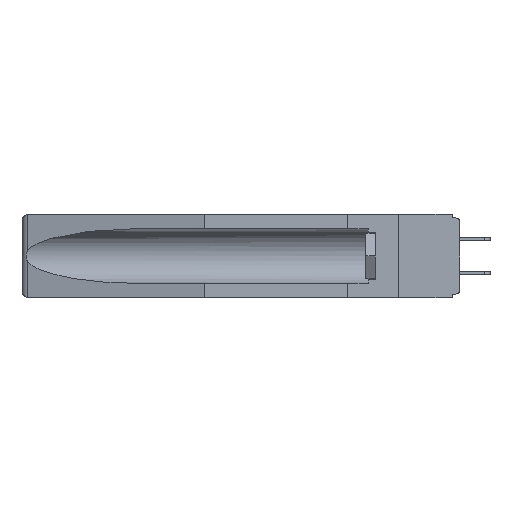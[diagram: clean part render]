
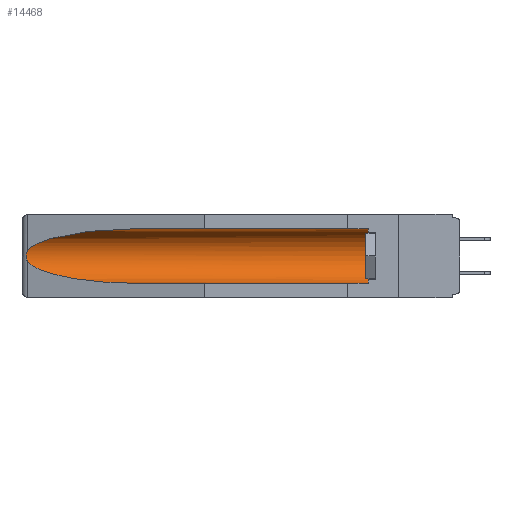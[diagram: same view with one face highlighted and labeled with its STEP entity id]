
A CAD part, left-side view. The second image highlights one B-rep face of the part: STEP entity #14468.
In plain terms, the highlighted cylindrical face has radius 2.857 mm (diameter 5.715 mm), a partial arc.
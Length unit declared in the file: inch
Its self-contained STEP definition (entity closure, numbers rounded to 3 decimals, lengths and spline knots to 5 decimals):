
#339 = DIRECTION ( 'NONE',  ( 0., 1., 0. ) ) ;
#599 = EDGE_CURVE ( 'NONE', #6788, #26495, #5344, .T. ) ;
#1136 = CARTESIAN_POINT ( 'NONE',  ( 0.26537, 1.52718, -0.14972 ) ) ;
#2429 = VERTEX_POINT ( 'NONE', #30584 ) ;
#2439 = CARTESIAN_POINT ( 'NONE',  ( 0.155, -0.30754, -0.1715 ) ) ;
#2625 = CARTESIAN_POINT ( 'NONE',  ( 0.155, 0.126, -0.284 ) ) ;
#2867 = EDGE_CURVE ( 'NONE', #6788, #27530, #25446, .T. ) ;
#3631 = CYLINDRICAL_SURFACE ( 'NONE', #12495, 0.1125 ) ;
#4222 = ORIENTED_EDGE ( 'NONE', *, *, #30629, .T. ) ;
#5344 = LINE ( 'NONE', #17203, #15651 ) ;
#5813 = CARTESIAN_POINT ( 'NONE',  ( 0.155, 1.07973, -0.059 ) ) ;
#6539 = ORIENTED_EDGE ( 'NONE', *, *, #599, .F. ) ;
#6788 = VERTEX_POINT ( 'NONE', #2625 ) ;
#6806 = CARTESIAN_POINT ( 'NONE',  ( 0.2673, 1.5327, -0.16383 ) ) ;
#7221 = CARTESIAN_POINT ( 'NONE',  ( 0.2675, 1.53308, -0.16763 ) ) ;
#7276 = B_SPLINE_CURVE_WITH_KNOTS ( 'NONE', 3,
 ( #19146, #23837, #26482, #6806, #7221, #9262, #26268, #31126, #19249, #16601 ),
 .UNSPECIFIED., .F., .F.,
 ( 4, 2, 2, 2, 4 ),
 ( 0., 0.00029, 0.00058, 0.00087, 0.00117 ),
 .UNSPECIFIED. ) ;
#9235 =( BOUNDED_CURVE ( )  B_SPLINE_CURVE ( 3, ( #27372, #24932, #22724, #1136 ),
 .UNSPECIFIED., .F., .F. ) 
 B_SPLINE_CURVE_WITH_KNOTS ( ( 4, 4 ),
 ( 4.71239, 6.08839 ),
 .UNSPECIFIED. ) 
 CURVE ( )  GEOMETRIC_REPRESENTATION_ITEM ( )  RATIONAL_B_SPLINE_CURVE ( ( 1., 0.848, 0.848, 1. ) ) 
 REPRESENTATION_ITEM ( '' )  );
#9262 = CARTESIAN_POINT ( 'NONE',  ( 0.2675, 1.53308, -0.17534 ) ) ;
#9343 = CARTESIAN_POINT ( 'NONE',  ( 0.26537, 1.52718, -0.19328 ) ) ;
#10529 = EDGE_CURVE ( 'NONE', #27530, #24816, #23287, .T. ) ;
#12412 = DIRECTION ( 'NONE',  ( 0., 1., 0. ) ) ;
#12495 = AXIS2_PLACEMENT_3D ( 'NONE', #2439, #15195, #29806 ) ;
#12654 = CARTESIAN_POINT ( 'NONE',  ( 0.155, -0.30754, -0.059 ) ) ;
#12719 = EDGE_CURVE ( 'NONE', #2429, #30623, #7276, .T. ) ;
#13387 = DIRECTION ( 'NONE',  ( 0., -1., 0. ) ) ;
#13580 = ORIENTED_EDGE ( 'NONE', *, *, #10529, .T. ) ;
#14223 = CARTESIAN_POINT ( 'NONE',  ( 0.25451, 1.48313, -0.24835 ) ) ;
#14468 = ADVANCED_FACE ( 'NONE', ( #14656 ), #3631, .F. ) ;
#14656 = FACE_OUTER_BOUND ( 'NONE', #26239, .T. ) ;
#15195 = DIRECTION ( 'NONE',  ( 0., 1., 0. ) ) ;
#15651 = VECTOR ( 'NONE', #12412, 39.37008 ) ;
#16601 = CARTESIAN_POINT ( 'NONE',  ( 0.26537, 1.52718, -0.19328 ) ) ;
#17203 = CARTESIAN_POINT ( 'NONE',  ( 0.155, -0.30754, -0.284 ) ) ;
#18213 =( BOUNDED_CURVE ( )  B_SPLINE_CURVE ( 3, ( #9343, #14223, #30993, #23604 ),
 .UNSPECIFIED., .F., .F. ) 
 B_SPLINE_CURVE_WITH_KNOTS ( ( 4, 4 ),
 ( 0.1948, 1.5708 ),
 .UNSPECIFIED. ) 
 CURVE ( )  GEOMETRIC_REPRESENTATION_ITEM ( )  RATIONAL_B_SPLINE_CURVE ( ( 1., 0.848, 0.848, 1. ) ) 
 REPRESENTATION_ITEM ( '' )  );
#19146 = CARTESIAN_POINT ( 'NONE',  ( 0.26537, 1.52718, -0.14972 ) ) ;
#19249 = CARTESIAN_POINT ( 'NONE',  ( 0.26597, 1.5296, -0.19026 ) ) ;
#19621 = ORIENTED_EDGE ( 'NONE', *, *, #2867, .T. ) ;
#20356 = EDGE_CURVE ( 'NONE', #24816, #2429, #9235, .T. ) ;
#20515 = CARTESIAN_POINT ( 'NONE',  ( 0.155, 0.126, -0.1715 ) ) ;
#20977 = VECTOR ( 'NONE', #339, 39.37008 ) ;
#22131 = ORIENTED_EDGE ( 'NONE', *, *, #20356, .T. ) ;
#22724 = CARTESIAN_POINT ( 'NONE',  ( 0.25451, 1.48313, -0.09465 ) ) ;
#23287 = LINE ( 'NONE', #12654, #20977 ) ;
#23604 = CARTESIAN_POINT ( 'NONE',  ( 0.155, 1.07973, -0.284 ) ) ;
#23837 = CARTESIAN_POINT ( 'NONE',  ( 0.26597, 1.52961, -0.15275 ) ) ;
#24465 = CARTESIAN_POINT ( 'NONE',  ( 0.155, 1.07973, -0.284 ) ) ;
#24816 = VERTEX_POINT ( 'NONE', #5813 ) ;
#24932 = CARTESIAN_POINT ( 'NONE',  ( 0.21114, 1.30732, -0.059 ) ) ;
#25446 = CIRCLE ( 'NONE', #26332, 0.1125 ) ;
#25507 = DIRECTION ( 'NONE',  ( 0., 0., 1. ) ) ;
#26239 = EDGE_LOOP ( 'NONE', ( #22131, #30837, #4222, #6539, #19621, #13580 ) ) ;
#26268 = CARTESIAN_POINT ( 'NONE',  ( 0.2673, 1.53269, -0.17917 ) ) ;
#26332 = AXIS2_PLACEMENT_3D ( 'NONE', #20515, #13387, #25507 ) ;
#26482 = CARTESIAN_POINT ( 'NONE',  ( 0.26654, 1.53092, -0.15636 ) ) ;
#26495 = VERTEX_POINT ( 'NONE', #24465 ) ;
#27372 = CARTESIAN_POINT ( 'NONE',  ( 0.155, 1.07973, -0.059 ) ) ;
#27530 = VERTEX_POINT ( 'NONE', #30566 ) ;
#29806 = DIRECTION ( 'NONE',  ( 0., 0., 1. ) ) ;
#30566 = CARTESIAN_POINT ( 'NONE',  ( 0.155, 0.126, -0.059 ) ) ;
#30584 = CARTESIAN_POINT ( 'NONE',  ( 0.26537, 1.52718, -0.14972 ) ) ;
#30623 = VERTEX_POINT ( 'NONE', #31201 ) ;
#30629 = EDGE_CURVE ( 'NONE', #30623, #26495, #18213, .T. ) ;
#30837 = ORIENTED_EDGE ( 'NONE', *, *, #12719, .T. ) ;
#30993 = CARTESIAN_POINT ( 'NONE',  ( 0.21114, 1.30732, -0.284 ) ) ;
#31126 = CARTESIAN_POINT ( 'NONE',  ( 0.26655, 1.53094, -0.18657 ) ) ;
#31201 = CARTESIAN_POINT ( 'NONE',  ( 0.26537, 1.52718, -0.19328 ) ) ;
